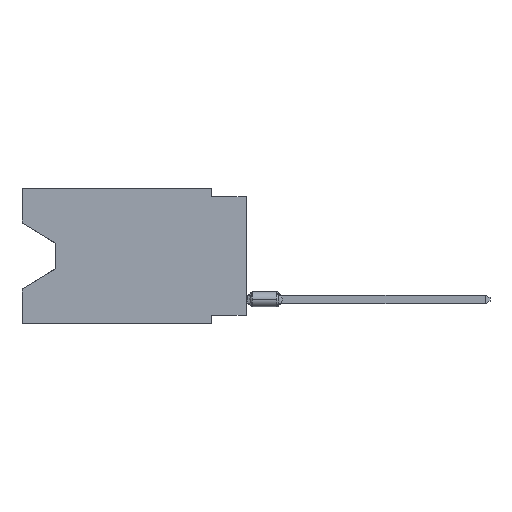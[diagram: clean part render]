
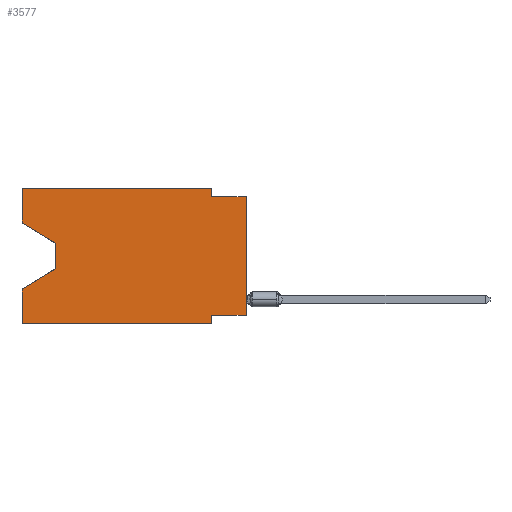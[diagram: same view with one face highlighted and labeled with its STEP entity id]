
A CAD part, left-side view. The second image highlights one B-rep face of the part: STEP entity #3577.
In plain terms, the highlighted planar face has unit normal (-1, 0, 0).
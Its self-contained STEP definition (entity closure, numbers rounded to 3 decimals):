
#5 = LINE ( 'NONE', #260, #13800 ) ;
#96 = ORIENTED_EDGE ( 'NONE', *, *, #1187, .F. ) ;
#260 = CARTESIAN_POINT ( 'NONE',  ( 0., 2.54, -9.906 ) ) ;
#326 = DIRECTION ( 'NONE',  ( 0., -1., 0. ) ) ;
#758 = LINE ( 'NONE', #5946, #5051 ) ;
#1187 = EDGE_CURVE ( 'NONE', #15221, #15778, #5, .T. ) ;
#1285 = VERTEX_POINT ( 'NONE', #4590 ) ;
#1447 = EDGE_CURVE ( 'NONE', #1841, #5470, #758, .T. ) ;
#1615 = LINE ( 'NONE', #15639, #3186 ) ;
#1688 = VERTEX_POINT ( 'NONE', #6558 ) ;
#1841 = VERTEX_POINT ( 'NONE', #13660 ) ;
#1893 = VECTOR ( 'NONE', #12614, 1000. ) ;
#2120 = EDGE_CURVE ( 'NONE', #12716, #15221, #6871, .T. ) ;
#2254 = VECTOR ( 'NONE', #10725, 1000. ) ;
#2545 = VECTOR ( 'NONE', #13961, 1000. ) ;
#2578 = LINE ( 'NONE', #11646, #14014 ) ;
#2666 = DIRECTION ( 'NONE',  ( 0., 0., 1. ) ) ;
#2783 = VERTEX_POINT ( 'NONE', #15760 ) ;
#3137 = VECTOR ( 'NONE', #15852, 1000. ) ;
#3186 = VECTOR ( 'NONE', #326, 1000. ) ;
#3577 = ADVANCED_FACE ( 'NONE', ( #12089 ), #6778, .F. ) ;
#3643 = EDGE_CURVE ( 'NONE', #4568, #1285, #14496, .T. ) ;
#3849 = ORIENTED_EDGE ( 'NONE', *, *, #1447, .T. ) ;
#4040 = CARTESIAN_POINT ( 'NONE',  ( 0., 16.383, 0. ) ) ;
#4098 = CARTESIAN_POINT ( 'NONE',  ( 0., 2.54, 0. ) ) ;
#4221 = DIRECTION ( 'NONE',  ( 0., 1., 0. ) ) ;
#4241 = CARTESIAN_POINT ( 'NONE',  ( 0., 16.383, -2.546 ) ) ;
#4313 = ORIENTED_EDGE ( 'NONE', *, *, #12201, .T. ) ;
#4499 = VERTEX_POINT ( 'NONE', #15576 ) ;
#4568 = VERTEX_POINT ( 'NONE', #15188 ) ;
#4590 = CARTESIAN_POINT ( 'NONE',  ( 0., 2.54, 0. ) ) ;
#5040 = VECTOR ( 'NONE', #7316, 1000. ) ;
#5051 = VECTOR ( 'NONE', #9892, 1000. ) ;
#5283 = CARTESIAN_POINT ( 'NONE',  ( 0., 16.383, -9.906 ) ) ;
#5399 = DIRECTION ( 'NONE',  ( 0., 0., -1. ) ) ;
#5470 = VERTEX_POINT ( 'NONE', #9274 ) ;
#5874 = EDGE_CURVE ( 'NONE', #1285, #1688, #16027, .T. ) ;
#5946 = CARTESIAN_POINT ( 'NONE',  ( 0., 13.97, -4.013 ) ) ;
#6558 = CARTESIAN_POINT ( 'NONE',  ( 0., 2.54, -0.635 ) ) ;
#6660 = EDGE_CURVE ( 'NONE', #15627, #15778, #1615, .T. ) ;
#6694 = DIRECTION ( 'NONE',  ( 1., 0., 0. ) ) ;
#6753 = CARTESIAN_POINT ( 'NONE',  ( 0., 0., 0. ) ) ;
#6778 = PLANE ( 'NONE',  #14287 ) ;
#6871 = LINE ( 'NONE', #15969, #10001 ) ;
#6892 = ORIENTED_EDGE ( 'NONE', *, *, #13376, .T. ) ;
#7316 = DIRECTION ( 'NONE',  ( 0., 0., 1. ) ) ;
#7395 = LINE ( 'NONE', #8851, #1893 ) ;
#7403 = DIRECTION ( 'NONE',  ( 0., -1., 0. ) ) ;
#7521 = EDGE_LOOP ( 'NONE', ( #6892, #3849, #4313, #12351, #10629, #96, #15150, #8784, #13130, #11887, #12771, #10355 ) ) ;
#7789 = VERTEX_POINT ( 'NONE', #4241 ) ;
#7979 = CARTESIAN_POINT ( 'NONE',  ( 0., 16.383, 0. ) ) ;
#8039 = LINE ( 'NONE', #6753, #5040 ) ;
#8647 = DIRECTION ( 'NONE',  ( 0., 0., 1. ) ) ;
#8784 = ORIENTED_EDGE ( 'NONE', *, *, #15752, .T. ) ;
#8816 = LINE ( 'NONE', #12670, #12656 ) ;
#8851 = CARTESIAN_POINT ( 'NONE',  ( 0., 16.383, -2.546 ) ) ;
#9274 = CARTESIAN_POINT ( 'NONE',  ( 0., 13.97, -5.893 ) ) ;
#9892 = DIRECTION ( 'NONE',  ( 0., 0., -1. ) ) ;
#10001 = VECTOR ( 'NONE', #4221, 1000. ) ;
#10062 = LINE ( 'NONE', #13832, #10383 ) ;
#10302 = EDGE_CURVE ( 'NONE', #1688, #2783, #10062, .T. ) ;
#10355 = ORIENTED_EDGE ( 'NONE', *, *, #12219, .F. ) ;
#10383 = VECTOR ( 'NONE', #7403, 1000. ) ;
#10629 = ORIENTED_EDGE ( 'NONE', *, *, #6660, .T. ) ;
#10691 = DIRECTION ( 'NONE',  ( 0., 0., -1. ) ) ;
#10725 = DIRECTION ( 'NONE',  ( 0., -1., 0. ) ) ;
#10872 = CARTESIAN_POINT ( 'NONE',  ( 0., 2.54, -9.906 ) ) ;
#11646 = CARTESIAN_POINT ( 'NONE',  ( 0., 16.383, 0. ) ) ;
#11887 = ORIENTED_EDGE ( 'NONE', *, *, #5874, .F. ) ;
#12089 = FACE_OUTER_BOUND ( 'NONE', #7521, .T. ) ;
#12201 = EDGE_CURVE ( 'NONE', #5470, #4499, #16629, .T. ) ;
#12219 = EDGE_CURVE ( 'NONE', #7789, #4568, #8816, .T. ) ;
#12351 = ORIENTED_EDGE ( 'NONE', *, *, #12358, .F. ) ;
#12358 = EDGE_CURVE ( 'NONE', #15627, #4499, #2578, .T. ) ;
#12614 = DIRECTION ( 'NONE',  ( 0., -0.855, -0.519 ) ) ;
#12656 = VECTOR ( 'NONE', #8647, 1000. ) ;
#12670 = CARTESIAN_POINT ( 'NONE',  ( 0., 16.383, 0. ) ) ;
#12716 = VERTEX_POINT ( 'NONE', #16158 ) ;
#12771 = ORIENTED_EDGE ( 'NONE', *, *, #3643, .F. ) ;
#12844 = CARTESIAN_POINT ( 'NONE',  ( 0., 13.97, -5.893 ) ) ;
#13130 = ORIENTED_EDGE ( 'NONE', *, *, #10302, .F. ) ;
#13376 = EDGE_CURVE ( 'NONE', #7789, #1841, #7395, .T. ) ;
#13660 = CARTESIAN_POINT ( 'NONE',  ( 0., 13.97, -4.013 ) ) ;
#13800 = VECTOR ( 'NONE', #10691, 1000. ) ;
#13832 = CARTESIAN_POINT ( 'NONE',  ( 0., 0., -0.635 ) ) ;
#13961 = DIRECTION ( 'NONE',  ( 0., 0.855, -0.519 ) ) ;
#14014 = VECTOR ( 'NONE', #2666, 1000. ) ;
#14287 = AXIS2_PLACEMENT_3D ( 'NONE', #4040, #6694, #5399 ) ;
#14496 = LINE ( 'NONE', #7979, #2254 ) ;
#15150 = ORIENTED_EDGE ( 'NONE', *, *, #2120, .F. ) ;
#15188 = CARTESIAN_POINT ( 'NONE',  ( 0., 16.383, 0. ) ) ;
#15221 = VERTEX_POINT ( 'NONE', #15864 ) ;
#15576 = CARTESIAN_POINT ( 'NONE',  ( 0., 16.383, -7.36 ) ) ;
#15627 = VERTEX_POINT ( 'NONE', #5283 ) ;
#15639 = CARTESIAN_POINT ( 'NONE',  ( 0., 16.383, -9.906 ) ) ;
#15752 = EDGE_CURVE ( 'NONE', #12716, #2783, #8039, .T. ) ;
#15760 = CARTESIAN_POINT ( 'NONE',  ( 0., 0., -0.635 ) ) ;
#15778 = VERTEX_POINT ( 'NONE', #10872 ) ;
#15852 = DIRECTION ( 'NONE',  ( 0., 0., -1. ) ) ;
#15864 = CARTESIAN_POINT ( 'NONE',  ( 0., 2.54, -9.271 ) ) ;
#15969 = CARTESIAN_POINT ( 'NONE',  ( 0., 0., -9.271 ) ) ;
#16027 = LINE ( 'NONE', #4098, #3137 ) ;
#16158 = CARTESIAN_POINT ( 'NONE',  ( 0., 0., -9.271 ) ) ;
#16629 = LINE ( 'NONE', #12844, #2545 ) ;
